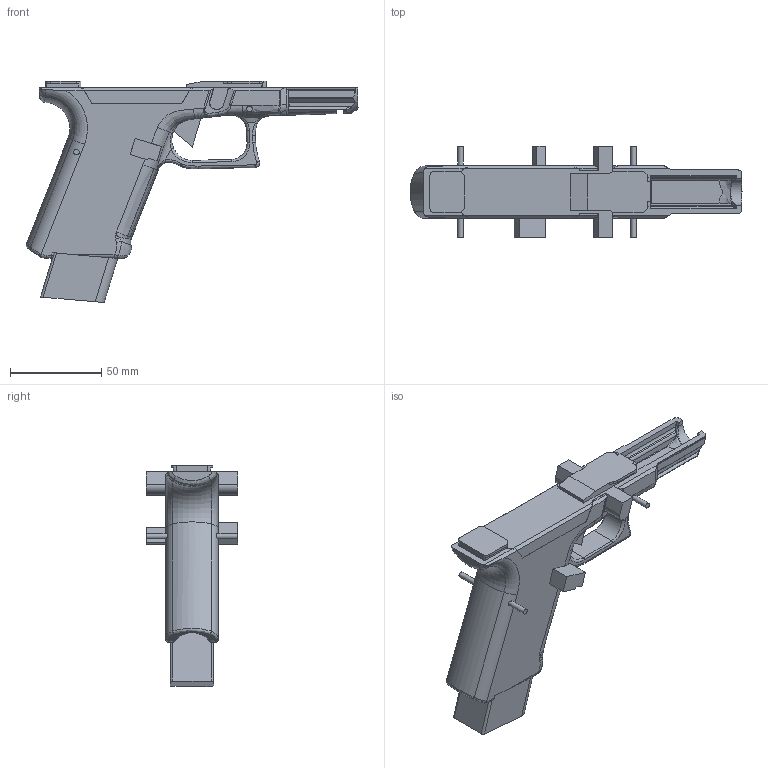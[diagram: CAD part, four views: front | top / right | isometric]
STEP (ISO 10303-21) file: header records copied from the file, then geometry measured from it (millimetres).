
FILE_DESCRIPTION(/* description */ (''),/* implementation_level */ '2;1');
FILE_NAME(/* name */ '120R Boolean Negative.step',/* time_stamp */ '2024-07-06T17:49:15-05:00',/* author */ (''),/* organization */ (''),/* preprocessor_version */ 'ST-DEVELOPER v20',/* originating_system */ 'Autodesk Translation Framework v13.14.0.145',/* authorisation */ '');
FILE_SCHEMA (('AUTOMOTIVE_DESIGN { 1 0 10303 214 3 1 1 }'));
Length unit declared in the file: millimetre
Products named in the file (5): 120G Compact; 120G Compact - Standard; X9-C (G19) RC1; Boolean V2 v6; RevE Boolean v1
Assembly tree (4 placements, depth 3):
  120G Compact
    120G Compact - Standard
      X9-C (G19) RC1
    Boolean V2 v6
      RevE Boolean v1
Bounding box: 182.13 x 50 x 121.31 mm (x, y, z)
Volume: 212029.1 mm3; surface area: 64941.5 mm2
Topology: 2 solids, 2 shells, 691 faces, 2102 edges, 1395 vertices
Faces by surface type: plane 301, bspline 209, cylinder 150, torus 16, cone 13, sphere 2
Full cylindrical faces by diameter (mm): 1.321 x2, 3 x8
Entity records: 47169 total; most frequent: CARTESIAN_POINT 29589, ORIENTED_EDGE 4176, DIRECTION 3011, EDGE_CURVE 2088, VERTEX_POINT 1396, AXIS2_PLACEMENT_3D 1015, LINE 981, VECTOR 981
